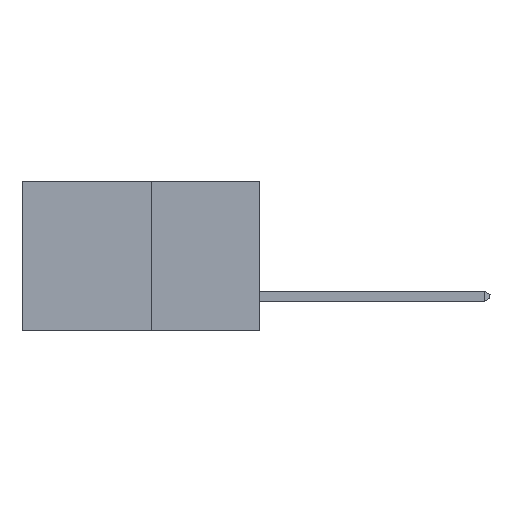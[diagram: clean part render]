
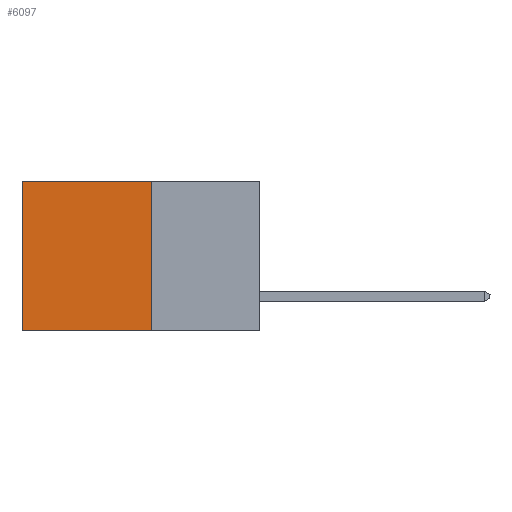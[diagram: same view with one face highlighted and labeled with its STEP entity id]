
A CAD part, left-side view. The second image highlights one B-rep face of the part: STEP entity #6097.
In plain terms, the highlighted planar face has unit normal (-1, 0, 0).
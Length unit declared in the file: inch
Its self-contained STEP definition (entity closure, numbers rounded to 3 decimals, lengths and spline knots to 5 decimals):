
#547 = DIRECTION ( 'NONE',  ( 0., 0., -1. ) ) ;
#667 = ORIENTED_EDGE ( 'NONE', *, *, #2135, .T. ) ;
#691 = ORIENTED_EDGE ( 'NONE', *, *, #12409, .F. ) ;
#797 = ORIENTED_EDGE ( 'NONE', *, *, #9366, .F. ) ;
#878 = ORIENTED_EDGE ( 'NONE', *, *, #2780, .T. ) ;
#1006 = CARTESIAN_POINT ( 'NONE',  ( 0.277, 0.27, -0.37 ) ) ;
#1184 = CARTESIAN_POINT ( 'NONE',  ( 0.277, 0.27, 0. ) ) ;
#1362 = LINE ( 'NONE', #1873, #6142 ) ;
#1368 = AXIS2_PLACEMENT_3D ( 'NONE', #6948, #6880, #6876 ) ;
#1579 = CARTESIAN_POINT ( 'NONE',  ( 0.277, 0.27, -0.37 ) ) ;
#1873 = CARTESIAN_POINT ( 'NONE',  ( 0.277, 0.27, -0.37 ) ) ;
#2135 = EDGE_CURVE ( 'NONE', #3662, #3247, #6168, .T. ) ;
#2780 = EDGE_CURVE ( 'NONE', #8614, #3662, #8347, .T. ) ;
#2974 = DIRECTION ( 'NONE',  ( 0., 0., -1. ) ) ;
#3154 = EDGE_LOOP ( 'NONE', ( #667, #691, #797, #878 ) ) ;
#3247 = VERTEX_POINT ( 'NONE', #7784 ) ;
#3561 = VECTOR ( 'NONE', #547, 39.37008 ) ;
#3562 = VECTOR ( 'NONE', #4014, 39.37008 ) ;
#3662 = VERTEX_POINT ( 'NONE', #5974 ) ;
#4014 = DIRECTION ( 'NONE',  ( 0., 1., 0. ) ) ;
#5813 = FACE_OUTER_BOUND ( 'NONE', #3154, .T. ) ;
#5974 = CARTESIAN_POINT ( 'NONE',  ( 0.277, 0.59, 0. ) ) ;
#6096 = DIRECTION ( 'NONE',  ( 0., 1., 0. ) ) ;
#6097 = ADVANCED_FACE ( 'NONE', ( #5813 ), #6933, .F. ) ;
#6142 = VECTOR ( 'NONE', #2974, 39.37008 ) ;
#6168 = LINE ( 'NONE', #9853, #3561 ) ;
#6876 = DIRECTION ( 'NONE',  ( 0., 0., -1. ) ) ;
#6880 = DIRECTION ( 'NONE',  ( 1., 0., 0. ) ) ;
#6933 = PLANE ( 'NONE',  #1368 ) ;
#6948 = CARTESIAN_POINT ( 'NONE',  ( 0.277, 0.27, -0.37 ) ) ;
#7784 = CARTESIAN_POINT ( 'NONE',  ( 0.277, 0.59, -0.37 ) ) ;
#8347 = LINE ( 'NONE', #1184, #3562 ) ;
#8614 = VERTEX_POINT ( 'NONE', #12390 ) ;
#8932 = LINE ( 'NONE', #1006, #11436 ) ;
#9366 = EDGE_CURVE ( 'NONE', #8614, #9814, #1362, .T. ) ;
#9814 = VERTEX_POINT ( 'NONE', #1579 ) ;
#9853 = CARTESIAN_POINT ( 'NONE',  ( 0.277, 0.59, -0.37 ) ) ;
#11436 = VECTOR ( 'NONE', #6096, 39.37008 ) ;
#12390 = CARTESIAN_POINT ( 'NONE',  ( 0.277, 0.27, 0. ) ) ;
#12409 = EDGE_CURVE ( 'NONE', #9814, #3247, #8932, .T. ) ;
